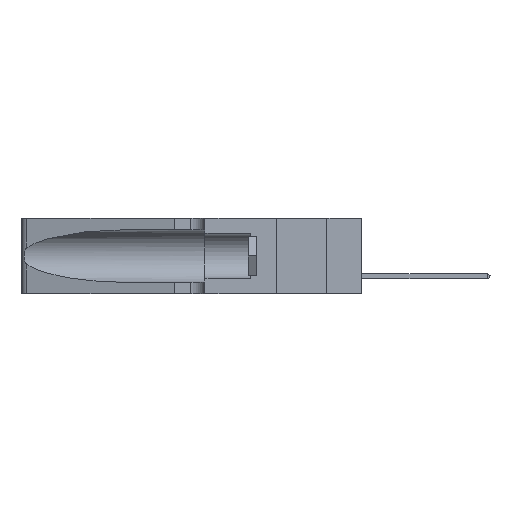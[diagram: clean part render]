
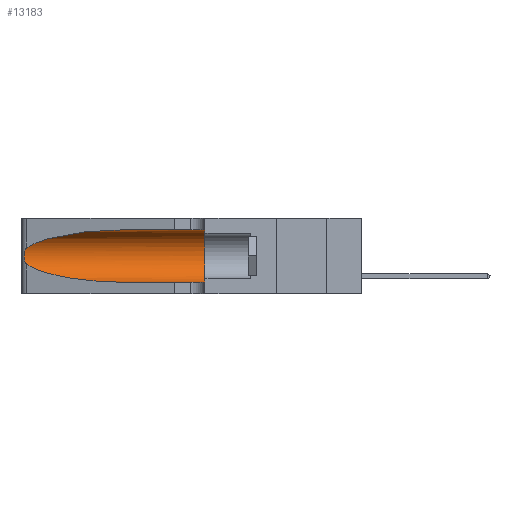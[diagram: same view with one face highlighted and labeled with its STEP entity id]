
A CAD part, left-side view. The second image highlights one B-rep face of the part: STEP entity #13183.
In plain terms, the highlighted cylindrical face has radius 3.308 mm (diameter 6.617 mm), a partial arc.
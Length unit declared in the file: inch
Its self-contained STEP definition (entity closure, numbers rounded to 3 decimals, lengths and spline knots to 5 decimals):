
#164 = ORIENTED_EDGE ( 'NONE', *, *, #24863, .T. ) ;
#727 = CARTESIAN_POINT ( 'NONE',  ( 0.1305, 0.35, 0.185 ) ) ;
#808 = CARTESIAN_POINT ( 'NONE',  ( 0.25555, 1.22994, 0.2215 ) ) ;
#1140 = CARTESIAN_POINT ( 'NONE',  ( 0.25787, 1.23484, 0.2124 ) ) ;
#1319 = VERTEX_POINT ( 'NONE', #7460 ) ;
#1434 = CARTESIAN_POINT ( 'NONE',  ( 0.1305, 0.72297, 0.31525 ) ) ;
#2169 =( BOUNDED_CURVE ( )  B_SPLINE_CURVE ( 3, ( #1434, #34975, #23756, #11992 ),
 .UNSPECIFIED., .F., .T. ) 
 B_SPLINE_CURVE_WITH_KNOTS ( ( 4, 4 ),
 ( 1.5708, 2.84003 ),
 .UNSPECIFIED. ) 
 CURVE ( )  GEOMETRIC_REPRESENTATION_ITEM ( )  RATIONAL_B_SPLINE_CURVE ( ( 1., 0.87, 0.87, 1. ) ) 
 REPRESENTATION_ITEM ( '' )  );
#2541 = AXIS2_PLACEMENT_3D ( 'NONE', #727, #38552, #38885 ) ;
#2737 = VECTOR ( 'NONE', #42293, 39.37008 ) ;
#5549 = CARTESIAN_POINT ( 'NONE',  ( 0.1305, 0.35, 0.05475 ) ) ;
#6165 = DIRECTION ( 'NONE',  ( 0., -1., 0. ) ) ;
#6753 = ORIENTED_EDGE ( 'NONE', *, *, #22993, .T. ) ;
#7257 = CARTESIAN_POINT ( 'NONE',  ( 0.26075, 1.23896, 0.178 ) ) ;
#7460 = CARTESIAN_POINT ( 'NONE',  ( 0.25487, 1.22718, 0.14631 ) ) ;
#8057 = CARTESIAN_POINT ( 'NONE',  ( 0.25487, 1.22718, 0.14631 ) ) ;
#8334 = CARTESIAN_POINT ( 'NONE',  ( 0.1305, 0.72297, 0.05475 ) ) ;
#8464 = ORIENTED_EDGE ( 'NONE', *, *, #36835, .T. ) ;
#8825 = CARTESIAN_POINT ( 'NONE',  ( 0.25789, 1.23486, 0.15765 ) ) ;
#8951 = CARTESIAN_POINT ( 'NONE',  ( 0.1305, 1.61858, 0.31525 ) ) ;
#10401 = LINE ( 'NONE', #16288, #2737 ) ;
#11992 = CARTESIAN_POINT ( 'NONE',  ( 0.25487, 1.22718, 0.22369 ) ) ;
#12353 = DIRECTION ( 'NONE',  ( 0., -1., 0. ) ) ;
#12593 = FACE_OUTER_BOUND ( 'NONE', #30462, .T. ) ;
#13183 = ADVANCED_FACE ( 'NONE', ( #12593 ), #32595, .F. ) ;
#14460 = CARTESIAN_POINT ( 'NONE',  ( 0.26018, 1.23835, 0.19895 ) ) ;
#15460 = CARTESIAN_POINT ( 'NONE',  ( 0.25487, 1.22718, 0.22369 ) ) ;
#15882 = CARTESIAN_POINT ( 'NONE',  ( 0.26017, 1.23833, 0.17102 ) ) ;
#16288 = CARTESIAN_POINT ( 'NONE',  ( 0.1305, 1.61858, 0.05475 ) ) ;
#16438 = CARTESIAN_POINT ( 'NONE',  ( 0.25854, 1.2359, 0.20912 ) ) ;
#16614 = B_SPLINE_CURVE_WITH_KNOTS ( 'NONE', 3,
 ( #15460, #808, #42947, #1140, #16438, #14460, #25945, #7257, #15882, #27202, #8825, #39538, #25857, #19373 ),
 .UNSPECIFIED., .F., .F.,
 ( 4, 2, 2, 2, 2, 2, 4 ),
 ( 0., 0.00027, 0.00053, 0.00107, 0.0016, 0.00187, 0.00214 ),
 .UNSPECIFIED. ) ;
#17244 = VERTEX_POINT ( 'NONE', #27081 ) ;
#18463 = VERTEX_POINT ( 'NONE', #8334 ) ;
#18947 = ORIENTED_EDGE ( 'NONE', *, *, #27326, .F. ) ;
#19373 = CARTESIAN_POINT ( 'NONE',  ( 0.25487, 1.22718, 0.14631 ) ) ;
#20301 = VERTEX_POINT ( 'NONE', #5549 ) ;
#21033 = EDGE_CURVE ( 'NONE', #1319, #18463, #39243, .T. ) ;
#22463 = EDGE_CURVE ( 'NONE', #17244, #20301, #32754, .T. ) ;
#22993 = EDGE_CURVE ( 'NONE', #18463, #20301, #10401, .T. ) ;
#23269 = VECTOR ( 'NONE', #6165, 39.37008 ) ;
#23756 = CARTESIAN_POINT ( 'NONE',  ( 0.2373, 1.15595, 0.28018 ) ) ;
#24863 = EDGE_CURVE ( 'NONE', #29865, #36711, #2169, .T. ) ;
#25857 = CARTESIAN_POINT ( 'NONE',  ( 0.25555, 1.22993, 0.14849 ) ) ;
#25945 = CARTESIAN_POINT ( 'NONE',  ( 0.26075, 1.23896, 0.19203 ) ) ;
#26217 = AXIS2_PLACEMENT_3D ( 'NONE', #46545, #12353, #42954 ) ;
#27081 = CARTESIAN_POINT ( 'NONE',  ( 0.1305, 0.35, 0.31525 ) ) ;
#27202 = CARTESIAN_POINT ( 'NONE',  ( 0.25856, 1.23593, 0.16098 ) ) ;
#27326 = EDGE_CURVE ( 'NONE', #29865, #17244, #44581, .T. ) ;
#29865 = VERTEX_POINT ( 'NONE', #31508 ) ;
#30462 = EDGE_LOOP ( 'NONE', ( #164, #8464, #40309, #6753, #45421, #18947 ) ) ;
#31508 = CARTESIAN_POINT ( 'NONE',  ( 0.1305, 0.72297, 0.31525 ) ) ;
#32595 = CYLINDRICAL_SURFACE ( 'NONE', #26217, 0.13025 ) ;
#32754 = CIRCLE ( 'NONE', #2541, 0.13025 ) ;
#33894 = CARTESIAN_POINT ( 'NONE',  ( 0.25487, 1.22718, 0.22369 ) ) ;
#34484 = CARTESIAN_POINT ( 'NONE',  ( 0.2373, 1.15595, 0.08982 ) ) ;
#34975 = CARTESIAN_POINT ( 'NONE',  ( 0.18966, 0.96281, 0.31525 ) ) ;
#36711 = VERTEX_POINT ( 'NONE', #33894 ) ;
#36835 = EDGE_CURVE ( 'NONE', #36711, #1319, #16614, .T. ) ;
#38552 = DIRECTION ( 'NONE',  ( 0., 1., 0. ) ) ;
#38797 = CARTESIAN_POINT ( 'NONE',  ( 0.18966, 0.96281, 0.05475 ) ) ;
#38885 = DIRECTION ( 'NONE',  ( 0., 0., 1. ) ) ;
#39243 =( BOUNDED_CURVE ( )  B_SPLINE_CURVE ( 3, ( #8057, #34484, #38797, #46355 ),
 .UNSPECIFIED., .F., .F. ) 
 B_SPLINE_CURVE_WITH_KNOTS ( ( 4, 4 ),
 ( 3.44316, 4.71239 ),
 .UNSPECIFIED. ) 
 CURVE ( )  GEOMETRIC_REPRESENTATION_ITEM ( )  RATIONAL_B_SPLINE_CURVE ( ( 1., 0.87, 0.87, 1. ) ) 
 REPRESENTATION_ITEM ( '' )  );
#39538 = CARTESIAN_POINT ( 'NONE',  ( 0.25639, 1.23186, 0.15144 ) ) ;
#40309 = ORIENTED_EDGE ( 'NONE', *, *, #21033, .T. ) ;
#42293 = DIRECTION ( 'NONE',  ( 0., -1., 0. ) ) ;
#42947 = CARTESIAN_POINT ( 'NONE',  ( 0.25639, 1.23184, 0.21858 ) ) ;
#42954 = DIRECTION ( 'NONE',  ( 0., 0., -1. ) ) ;
#44581 = LINE ( 'NONE', #8951, #23269 ) ;
#45421 = ORIENTED_EDGE ( 'NONE', *, *, #22463, .F. ) ;
#46355 = CARTESIAN_POINT ( 'NONE',  ( 0.1305, 0.72297, 0.05475 ) ) ;
#46545 = CARTESIAN_POINT ( 'NONE',  ( 0.1305, 1.61858, 0.185 ) ) ;
